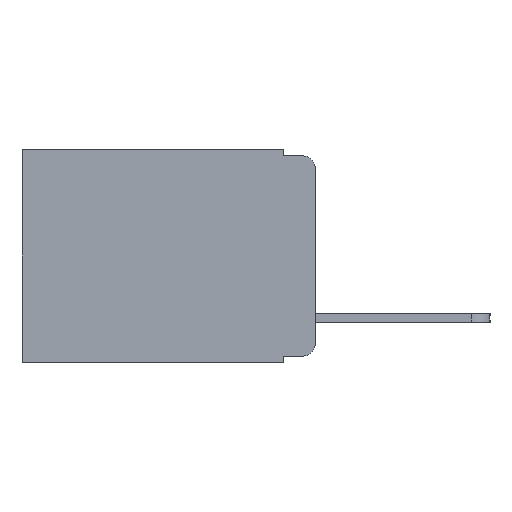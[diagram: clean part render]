
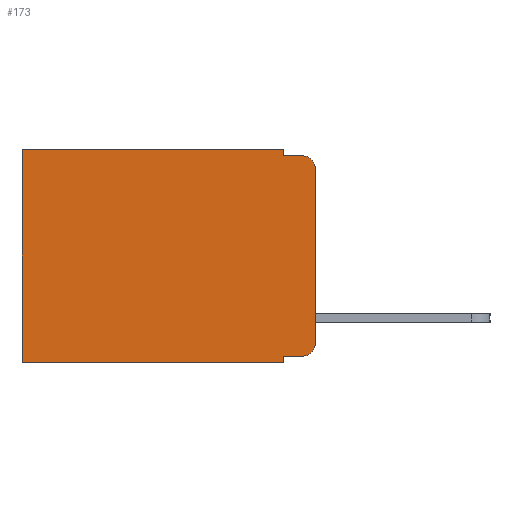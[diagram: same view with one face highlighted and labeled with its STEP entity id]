
A CAD part, left-side view. The second image highlights one B-rep face of the part: STEP entity #173.
In plain terms, the highlighted planar face has unit normal (-1, 0, 0).
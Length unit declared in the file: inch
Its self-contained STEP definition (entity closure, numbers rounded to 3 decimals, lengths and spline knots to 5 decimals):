
#8 = VERTEX_POINT ( 'NONE', #10726 ) ;
#72 = VERTEX_POINT ( 'NONE', #15588 ) ;
#173 = ADVANCED_FACE ( 'NONE', ( #10070 ), #17339, .F. ) ;
#660 = DIRECTION ( 'NONE',  ( 0., 0., -1. ) ) ;
#916 = VECTOR ( 'NONE', #17855, 39.37008 ) ;
#962 = ORIENTED_EDGE ( 'NONE', *, *, #15730, .T. ) ;
#1025 = VECTOR ( 'NONE', #4473, 39.37008 ) ;
#1230 = CARTESIAN_POINT ( 'NONE',  ( 0.298, 0.051, 0. ) ) ;
#1451 = CARTESIAN_POINT ( 'NONE',  ( 0.298, 0.051, -0.333 ) ) ;
#1485 = AXIS2_PLACEMENT_3D ( 'NONE', #8543, #8483, #3289 ) ;
#2133 = ORIENTED_EDGE ( 'NONE', *, *, #4605, .F. ) ;
#2492 = AXIS2_PLACEMENT_3D ( 'NONE', #17885, #9534, #660 ) ;
#2879 = ORIENTED_EDGE ( 'NONE', *, *, #16700, .F. ) ;
#2994 = DIRECTION ( 'NONE',  ( 0., -1., 0. ) ) ;
#3289 = DIRECTION ( 'NONE',  ( 0., 0., -1. ) ) ;
#3349 = ORIENTED_EDGE ( 'NONE', *, *, #15963, .T. ) ;
#3641 = CARTESIAN_POINT ( 'NONE',  ( 0.298, 0.051, 0. ) ) ;
#3715 = VERTEX_POINT ( 'NONE', #14089 ) ;
#3723 = EDGE_CURVE ( 'NONE', #13322, #11795, #12305, .T. ) ;
#3813 = LINE ( 'NONE', #10282, #11068 ) ;
#3913 = DIRECTION ( 'NONE',  ( 0., 0., -1. ) ) ;
#4426 = LINE ( 'NONE', #1451, #11678 ) ;
#4473 = DIRECTION ( 'NONE',  ( 0., 1., 0. ) ) ;
#4532 = CARTESIAN_POINT ( 'NONE',  ( 0.298, 0., 0. ) ) ;
#4605 = EDGE_CURVE ( 'NONE', #13322, #5235, #8962, .T. ) ;
#4837 = ORIENTED_EDGE ( 'NONE', *, *, #3723, .T. ) ;
#5001 = LINE ( 'NONE', #11692, #1025 ) ;
#5010 = VERTEX_POINT ( 'NONE', #5684 ) ;
#5235 = VERTEX_POINT ( 'NONE', #14972 ) ;
#5667 = LINE ( 'NONE', #8701, #15744 ) ;
#5684 = CARTESIAN_POINT ( 'NONE',  ( 0.298, 0.051, -0.343 ) ) ;
#6614 = CARTESIAN_POINT ( 'NONE',  ( 0.298, 0.473, 0. ) ) ;
#6738 = EDGE_CURVE ( 'NONE', #3715, #11795, #3813, .T. ) ;
#7251 = VECTOR ( 'NONE', #8076, 39.37008 ) ;
#7321 = CIRCLE ( 'NONE', #2492, 0.02 ) ;
#7491 = ORIENTED_EDGE ( 'NONE', *, *, #6738, .F. ) ;
#8076 = DIRECTION ( 'NONE',  ( 0., 0., -1. ) ) ;
#8483 = DIRECTION ( 'NONE',  ( -1., 0., 0. ) ) ;
#8543 = CARTESIAN_POINT ( 'NONE',  ( 0.298, 0.02, -0.03 ) ) ;
#8691 = CARTESIAN_POINT ( 'NONE',  ( 0.298, 0., -0.03 ) ) ;
#8701 = CARTESIAN_POINT ( 'NONE',  ( 0.298, 0., -0.343 ) ) ;
#8815 = LINE ( 'NONE', #10878, #916 ) ;
#8962 = LINE ( 'NONE', #4532, #12264 ) ;
#9411 = EDGE_LOOP ( 'NONE', ( #2133, #4837, #7491, #9751, #962, #12884, #2879, #16968, #11962, #3349 ) ) ;
#9534 = DIRECTION ( 'NONE',  ( -1., 0., 0. ) ) ;
#9545 = EDGE_CURVE ( 'NONE', #15080, #3715, #13950, .T. ) ;
#9751 = ORIENTED_EDGE ( 'NONE', *, *, #9545, .F. ) ;
#10070 = FACE_OUTER_BOUND ( 'NONE', #9411, .T. ) ;
#10282 = CARTESIAN_POINT ( 'NONE',  ( 0.298, 0.051, -0.01 ) ) ;
#10722 = EDGE_CURVE ( 'NONE', #8, #5010, #8815, .T. ) ;
#10726 = CARTESIAN_POINT ( 'NONE',  ( 0.298, 0.051, -0.333 ) ) ;
#10878 = CARTESIAN_POINT ( 'NONE',  ( 0.298, 0.051, 0. ) ) ;
#11068 = VECTOR ( 'NONE', #12536, 39.37008 ) ;
#11077 = CARTESIAN_POINT ( 'NONE',  ( 0.298, 0.02, -0.01 ) ) ;
#11107 = VERTEX_POINT ( 'NONE', #16569 ) ;
#11596 = VERTEX_POINT ( 'NONE', #16328 ) ;
#11678 = VECTOR ( 'NONE', #2994, 39.37008 ) ;
#11692 = CARTESIAN_POINT ( 'NONE',  ( 0.298, 0., 0. ) ) ;
#11745 = AXIS2_PLACEMENT_3D ( 'NONE', #17356, #17399, #17436 ) ;
#11795 = VERTEX_POINT ( 'NONE', #11077 ) ;
#11962 = ORIENTED_EDGE ( 'NONE', *, *, #18179, .T. ) ;
#12264 = VECTOR ( 'NONE', #3913, 39.37008 ) ;
#12305 = CIRCLE ( 'NONE', #1485, 0.02 ) ;
#12536 = DIRECTION ( 'NONE',  ( 0., -1., 0. ) ) ;
#12884 = ORIENTED_EDGE ( 'NONE', *, *, #17599, .T. ) ;
#13082 = VECTOR ( 'NONE', #16481, 39.37008 ) ;
#13322 = VERTEX_POINT ( 'NONE', #8691 ) ;
#13950 = LINE ( 'NONE', #3641, #13082 ) ;
#14089 = CARTESIAN_POINT ( 'NONE',  ( 0.298, 0.051, -0.01 ) ) ;
#14972 = CARTESIAN_POINT ( 'NONE',  ( 0.298, 0., -0.313 ) ) ;
#15080 = VERTEX_POINT ( 'NONE', #1230 ) ;
#15588 = CARTESIAN_POINT ( 'NONE',  ( 0.298, 0.473, 0. ) ) ;
#15730 = EDGE_CURVE ( 'NONE', #15080, #72, #5001, .T. ) ;
#15744 = VECTOR ( 'NONE', #17076, 39.37008 ) ;
#15963 = EDGE_CURVE ( 'NONE', #11596, #5235, #7321, .T. ) ;
#16328 = CARTESIAN_POINT ( 'NONE',  ( 0.298, 0.02, -0.333 ) ) ;
#16481 = DIRECTION ( 'NONE',  ( 0., 0., -1. ) ) ;
#16569 = CARTESIAN_POINT ( 'NONE',  ( 0.298, 0.473, -0.343 ) ) ;
#16700 = EDGE_CURVE ( 'NONE', #5010, #11107, #5667, .T. ) ;
#16968 = ORIENTED_EDGE ( 'NONE', *, *, #10722, .F. ) ;
#17076 = DIRECTION ( 'NONE',  ( 0., 1., 0. ) ) ;
#17339 = PLANE ( 'NONE',  #11745 ) ;
#17356 = CARTESIAN_POINT ( 'NONE',  ( 0.298, 0., 0. ) ) ;
#17399 = DIRECTION ( 'NONE',  ( 1., 0., 0. ) ) ;
#17436 = DIRECTION ( 'NONE',  ( 0., 0., -1. ) ) ;
#17599 = EDGE_CURVE ( 'NONE', #72, #11107, #18012, .T. ) ;
#17855 = DIRECTION ( 'NONE',  ( 0., 0., -1. ) ) ;
#17885 = CARTESIAN_POINT ( 'NONE',  ( 0.298, 0.02, -0.313 ) ) ;
#18012 = LINE ( 'NONE', #6614, #7251 ) ;
#18179 = EDGE_CURVE ( 'NONE', #8, #11596, #4426, .T. ) ;
